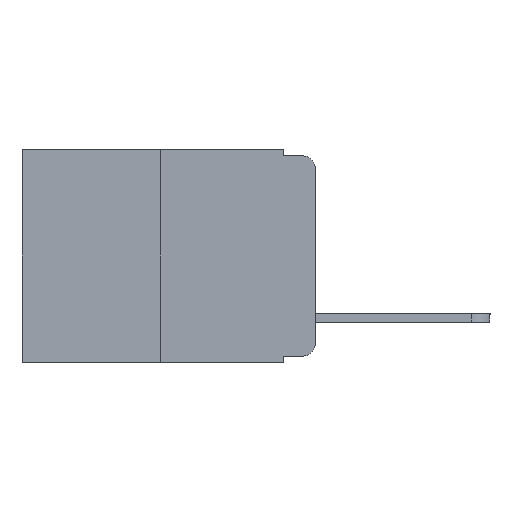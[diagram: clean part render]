
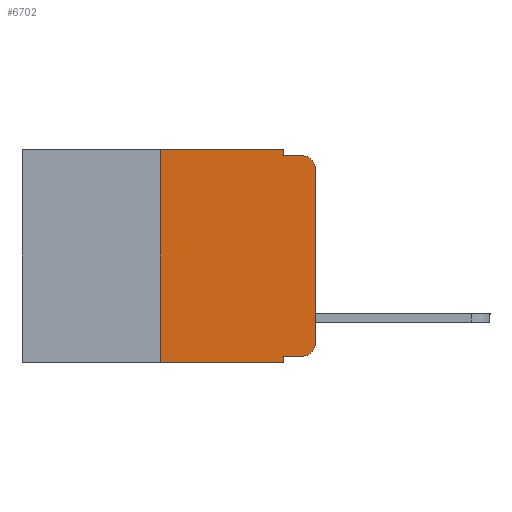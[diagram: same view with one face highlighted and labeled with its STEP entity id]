
A CAD part, left-side view. The second image highlights one B-rep face of the part: STEP entity #6702.
In plain terms, the highlighted planar face has unit normal (-1, 0, 0).
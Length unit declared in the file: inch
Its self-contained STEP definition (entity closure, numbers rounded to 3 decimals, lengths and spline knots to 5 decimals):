
#702 = VERTEX_POINT ( 'NONE', #15980 ) ;
#1122 = CARTESIAN_POINT ( 'NONE',  ( 0., 0.051, -0.01 ) ) ;
#1473 = VERTEX_POINT ( 'NONE', #17074 ) ;
#1486 = DIRECTION ( 'NONE',  ( 0., -1., 0. ) ) ;
#1575 = FACE_OUTER_BOUND ( 'NONE', #13837, .T. ) ;
#1655 = VECTOR ( 'NONE', #12483, 39.37008 ) ;
#1672 = CARTESIAN_POINT ( 'NONE',  ( 0., 0.473, -0.343 ) ) ;
#2061 = CARTESIAN_POINT ( 'NONE',  ( 0., 0.051, -0.343 ) ) ;
#2208 = AXIS2_PLACEMENT_3D ( 'NONE', #15367, #8118, #17977 ) ;
#2248 = ORIENTED_EDGE ( 'NONE', *, *, #7287, .T. ) ;
#2276 = VERTEX_POINT ( 'NONE', #11351 ) ;
#2409 = VERTEX_POINT ( 'NONE', #15537 ) ;
#2746 = CARTESIAN_POINT ( 'NONE',  ( 0., 0.02, -0.313 ) ) ;
#3000 = EDGE_CURVE ( 'NONE', #6978, #2409, #5686, .T. ) ;
#3069 = AXIS2_PLACEMENT_3D ( 'NONE', #17008, #8554, #18352 ) ;
#3290 = CARTESIAN_POINT ( 'NONE',  ( 0., 0.25, 0. ) ) ;
#3409 = VECTOR ( 'NONE', #6599, 39.37008 ) ;
#3456 = CARTESIAN_POINT ( 'NONE',  ( 0., 0., 0. ) ) ;
#4106 = ORIENTED_EDGE ( 'NONE', *, *, #16054, .F. ) ;
#4409 = DIRECTION ( 'NONE',  ( 0., 0., -1. ) ) ;
#4687 = LINE ( 'NONE', #19461, #18856 ) ;
#5129 = DIRECTION ( 'NONE',  ( 0., 0., 1. ) ) ;
#5227 = EDGE_CURVE ( 'NONE', #2409, #14510, #10394, .T. ) ;
#5560 = ORIENTED_EDGE ( 'NONE', *, *, #3000, .F. ) ;
#5686 = LINE ( 'NONE', #18187, #8543 ) ;
#6306 = VERTEX_POINT ( 'NONE', #3290 ) ;
#6413 = ORIENTED_EDGE ( 'NONE', *, *, #5227, .F. ) ;
#6414 = EDGE_CURVE ( 'NONE', #1473, #14510, #6969, .T. ) ;
#6599 = DIRECTION ( 'NONE',  ( 0., 0., -1. ) ) ;
#6650 = CARTESIAN_POINT ( 'NONE',  ( 0., 0.25, 0. ) ) ;
#6702 = ADVANCED_FACE ( 'NONE', ( #1575 ), #11094, .F. ) ;
#6969 = CIRCLE ( 'NONE', #3069, 0.02 ) ;
#6978 = VERTEX_POINT ( 'NONE', #18506 ) ;
#7287 = EDGE_CURVE ( 'NONE', #2276, #13334, #14000, .T. ) ;
#7541 = EDGE_CURVE ( 'NONE', #13334, #1473, #9844, .T. ) ;
#7547 = ORIENTED_EDGE ( 'NONE', *, *, #6414, .T. ) ;
#7919 = VECTOR ( 'NONE', #11423, 39.37008 ) ;
#8084 = EDGE_CURVE ( 'NONE', #14079, #8203, #16078, .T. ) ;
#8118 = DIRECTION ( 'NONE',  ( 1., 0., 0. ) ) ;
#8203 = VERTEX_POINT ( 'NONE', #2061 ) ;
#8289 = DIRECTION ( 'NONE',  ( 0., 0., 1. ) ) ;
#8543 = VECTOR ( 'NONE', #18138, 39.37008 ) ;
#8554 = DIRECTION ( 'NONE',  ( -1., 0., 0. ) ) ;
#9688 = CARTESIAN_POINT ( 'NONE',  ( 0., 0.051, 0. ) ) ;
#9844 = LINE ( 'NONE', #3456, #13349 ) ;
#9862 = ORIENTED_EDGE ( 'NONE', *, *, #7541, .T. ) ;
#10130 = ORIENTED_EDGE ( 'NONE', *, *, #10351, .T. ) ;
#10351 = EDGE_CURVE ( 'NONE', #702, #2276, #4687, .T. ) ;
#10394 = LINE ( 'NONE', #1122, #1655 ) ;
#11094 = PLANE ( 'NONE',  #2208 ) ;
#11351 = CARTESIAN_POINT ( 'NONE',  ( 0., 0.02, -0.333 ) ) ;
#11423 = DIRECTION ( 'NONE',  ( 0., -1., 0. ) ) ;
#11504 = LINE ( 'NONE', #6650, #14862 ) ;
#11733 = ORIENTED_EDGE ( 'NONE', *, *, #8084, .T. ) ;
#12429 = CARTESIAN_POINT ( 'NONE',  ( 0., 0.25, -0.343 ) ) ;
#12483 = DIRECTION ( 'NONE',  ( 0., -1., 0. ) ) ;
#12744 = ORIENTED_EDGE ( 'NONE', *, *, #19231, .F. ) ;
#13334 = VERTEX_POINT ( 'NONE', #19389 ) ;
#13349 = VECTOR ( 'NONE', #5129, 39.37008 ) ;
#13759 = DIRECTION ( 'NONE',  ( -1., 0., 0. ) ) ;
#13837 = EDGE_LOOP ( 'NONE', ( #9862, #7547, #6413, #5560, #12744, #18965, #11733, #4106, #10130, #2248 ) ) ;
#14000 = CIRCLE ( 'NONE', #15334, 0.02 ) ;
#14079 = VERTEX_POINT ( 'NONE', #12429 ) ;
#14439 = CARTESIAN_POINT ( 'NONE',  ( 0., 0.02, -0.01 ) ) ;
#14510 = VERTEX_POINT ( 'NONE', #14439 ) ;
#14862 = VECTOR ( 'NONE', #8289, 39.37008 ) ;
#15334 = AXIS2_PLACEMENT_3D ( 'NONE', #2746, #13759, #4409 ) ;
#15367 = CARTESIAN_POINT ( 'NONE',  ( 0., 0.473, 0. ) ) ;
#15537 = CARTESIAN_POINT ( 'NONE',  ( 0., 0.051, -0.01 ) ) ;
#15975 = CARTESIAN_POINT ( 'NONE',  ( 0., 0.473, 0. ) ) ;
#15980 = CARTESIAN_POINT ( 'NONE',  ( 0., 0.051, -0.333 ) ) ;
#16054 = EDGE_CURVE ( 'NONE', #702, #8203, #19097, .T. ) ;
#16078 = LINE ( 'NONE', #1672, #7919 ) ;
#16879 = EDGE_CURVE ( 'NONE', #14079, #6306, #11504, .T. ) ;
#17008 = CARTESIAN_POINT ( 'NONE',  ( 0., 0.02, -0.03 ) ) ;
#17074 = CARTESIAN_POINT ( 'NONE',  ( 0., 0., -0.03 ) ) ;
#17246 = DIRECTION ( 'NONE',  ( 0., -1., 0. ) ) ;
#17977 = DIRECTION ( 'NONE',  ( 0., 0., -1. ) ) ;
#18138 = DIRECTION ( 'NONE',  ( 0., 0., -1. ) ) ;
#18187 = CARTESIAN_POINT ( 'NONE',  ( 0., 0.051, 0. ) ) ;
#18352 = DIRECTION ( 'NONE',  ( 0., 0., -1. ) ) ;
#18473 = VECTOR ( 'NONE', #17246, 39.37008 ) ;
#18506 = CARTESIAN_POINT ( 'NONE',  ( 0., 0.051, 0. ) ) ;
#18856 = VECTOR ( 'NONE', #1486, 39.37008 ) ;
#18866 = LINE ( 'NONE', #15975, #18473 ) ;
#18965 = ORIENTED_EDGE ( 'NONE', *, *, #16879, .F. ) ;
#19097 = LINE ( 'NONE', #9688, #3409 ) ;
#19231 = EDGE_CURVE ( 'NONE', #6306, #6978, #18866, .T. ) ;
#19389 = CARTESIAN_POINT ( 'NONE',  ( 0., 0., -0.313 ) ) ;
#19461 = CARTESIAN_POINT ( 'NONE',  ( 0., 0.051, -0.333 ) ) ;
